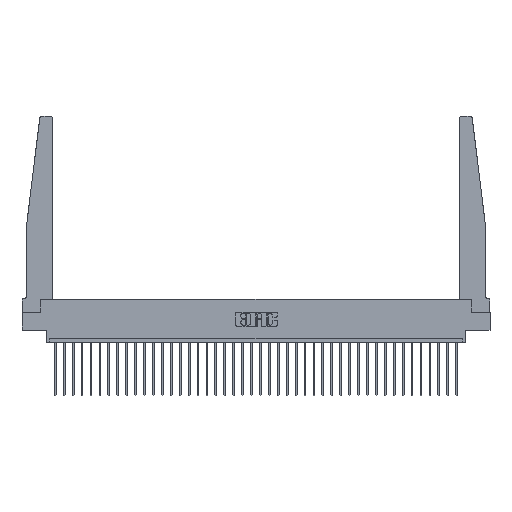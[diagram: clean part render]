
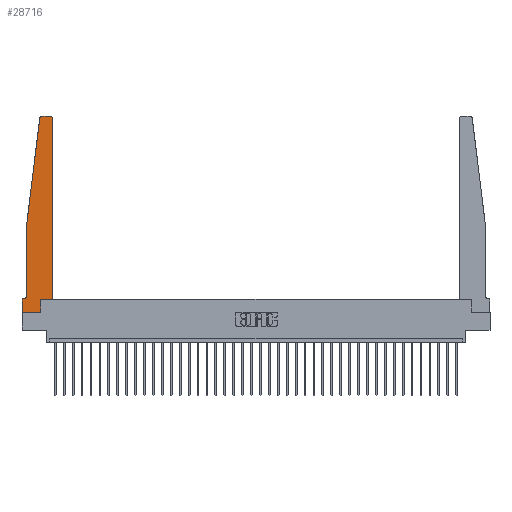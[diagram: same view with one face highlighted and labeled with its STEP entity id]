
A CAD part, top view. The second image highlights one B-rep face of the part: STEP entity #28716.
In plain terms, the highlighted planar face has unit normal (0, 0, 1).
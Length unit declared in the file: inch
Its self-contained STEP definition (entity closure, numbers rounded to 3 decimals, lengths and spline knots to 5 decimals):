
#335 = FACE_OUTER_BOUND ( 'NONE', #23905, .T. ) ;
#540 = AXIS2_PLACEMENT_3D ( 'NONE', #12960, #15313, #5533 ) ;
#733 = DIRECTION ( 'NONE',  ( 0., 0., 1. ) ) ;
#760 = CARTESIAN_POINT ( 'NONE',  ( 0.425, 2.72, 0.37 ) ) ;
#1057 = CIRCLE ( 'NONE', #30986, 0.03 ) ;
#1431 = LINE ( 'NONE', #20981, #18172 ) ;
#2554 = EDGE_CURVE ( 'NONE', #20029, #25679, #28582, .T. ) ;
#2625 = ORIENTED_EDGE ( 'NONE', *, *, #18938, .T. ) ;
#2832 = EDGE_CURVE ( 'NONE', #27348, #9803, #18638, .T. ) ;
#3004 = ORIENTED_EDGE ( 'NONE', *, *, #28220, .T. ) ;
#3468 = DIRECTION ( 'NONE',  ( 1., 0., 0. ) ) ;
#3637 = CARTESIAN_POINT ( 'NONE',  ( 0.27653, 2.72, 0.37 ) ) ;
#5130 = CARTESIAN_POINT ( 'NONE',  ( 0., 0., 0.37 ) ) ;
#5533 = DIRECTION ( 'NONE',  ( 1., 0., 0. ) ) ;
#5964 = CARTESIAN_POINT ( 'NONE',  ( 0.015, 0.1875, 0.37 ) ) ;
#6322 = LINE ( 'NONE', #21762, #27006 ) ;
#6409 = EDGE_CURVE ( 'NONE', #17926, #22845, #7710, .T. ) ;
#6859 = CARTESIAN_POINT ( 'NONE',  ( 0.425, 0.18, 0.37 ) ) ;
#7710 = LINE ( 'NONE', #22271, #25174 ) ;
#8232 = CARTESIAN_POINT ( 'NONE',  ( 0.065, 1.25, 0.37 ) ) ;
#9803 = VERTEX_POINT ( 'NONE', #13535 ) ;
#10226 = CARTESIAN_POINT ( 'NONE',  ( 0.065, 1.25, 0.37 ) ) ;
#10941 = AXIS2_PLACEMENT_3D ( 'NONE', #11388, #13925, #31398 ) ;
#11077 = CIRCLE ( 'NONE', #540, 0.03 ) ;
#11388 = CARTESIAN_POINT ( 'NONE',  ( 0., 0.1875, 0.37 ) ) ;
#11432 = VECTOR ( 'NONE', #13200, 39.37008 ) ;
#11489 = ORIENTED_EDGE ( 'NONE', *, *, #2554, .T. ) ;
#12028 = EDGE_CURVE ( 'NONE', #30605, #20029, #18039, .T. ) ;
#12380 = EDGE_CURVE ( 'NONE', #20665, #26768, #23200, .T. ) ;
#12960 = CARTESIAN_POINT ( 'NONE',  ( 0.395, 2.72, 0.37 ) ) ;
#13132 = CARTESIAN_POINT ( 'NONE',  ( 0.065, 0.2375, 0.37 ) ) ;
#13200 = DIRECTION ( 'NONE',  ( -0.122, -0.992, 0. ) ) ;
#13500 = PLANE ( 'NONE',  #10941 ) ;
#13535 = CARTESIAN_POINT ( 'NONE',  ( 0.2605, 0., 0.37 ) ) ;
#13925 = DIRECTION ( 'NONE',  ( 0., 0., 1. ) ) ;
#14068 = VERTEX_POINT ( 'NONE', #30506 ) ;
#14333 = ORIENTED_EDGE ( 'NONE', *, *, #16728, .T. ) ;
#14335 = AXIS2_PLACEMENT_3D ( 'NONE', #25271, #23043, #20587 ) ;
#15313 = DIRECTION ( 'NONE',  ( 0., 0., 1. ) ) ;
#15903 = ORIENTED_EDGE ( 'NONE', *, *, #17923, .T. ) ;
#16623 = CARTESIAN_POINT ( 'NONE',  ( 0.27653, 2.75, 0.37 ) ) ;
#16728 = EDGE_CURVE ( 'NONE', #25679, #22465, #11077, .T. ) ;
#17233 = VECTOR ( 'NONE', #28024, 39.37008 ) ;
#17825 = CIRCLE ( 'NONE', #14335, 0.05 ) ;
#17841 = VECTOR ( 'NONE', #3468, 39.37008 ) ;
#17923 = EDGE_CURVE ( 'NONE', #22465, #22476, #1431, .T. ) ;
#17926 = VERTEX_POINT ( 'NONE', #5964 ) ;
#18039 = LINE ( 'NONE', #6859, #18835 ) ;
#18124 = CARTESIAN_POINT ( 'NONE',  ( 0.065, 1.25, 0.37 ) ) ;
#18172 = VECTOR ( 'NONE', #21430, 39.37008 ) ;
#18638 = LINE ( 'NONE', #31359, #17841 ) ;
#18835 = VECTOR ( 'NONE', #24525, 39.37008 ) ;
#18938 = EDGE_CURVE ( 'NONE', #14068, #20665, #28979, .T. ) ;
#18998 = DIRECTION ( 'NONE',  ( 0., -1., 0. ) ) ;
#19973 = VECTOR ( 'NONE', #31827, 39.37008 ) ;
#20029 = VERTEX_POINT ( 'NONE', #23597 ) ;
#20587 = DIRECTION ( 'NONE',  ( -1., 0., 0. ) ) ;
#20665 = VERTEX_POINT ( 'NONE', #18124 ) ;
#20981 = CARTESIAN_POINT ( 'NONE',  ( 0.25, 2.75, 0.37 ) ) ;
#21056 = CARTESIAN_POINT ( 'NONE',  ( 0., 0.1875, 0.37 ) ) ;
#21094 = DIRECTION ( 'NONE',  ( 1., 0., 0. ) ) ;
#21430 = DIRECTION ( 'NONE',  ( -1., 0., 0. ) ) ;
#21583 = ORIENTED_EDGE ( 'NONE', *, *, #26490, .T. ) ;
#21728 = CARTESIAN_POINT ( 'NONE',  ( 0.395, 2.75, 0.37 ) ) ;
#21762 = CARTESIAN_POINT ( 'NONE',  ( 0., 0., 0.37 ) ) ;
#22271 = CARTESIAN_POINT ( 'NONE',  ( 0.065, 0.1875, 0.37 ) ) ;
#22465 = VERTEX_POINT ( 'NONE', #21728 ) ;
#22476 = VERTEX_POINT ( 'NONE', #16623 ) ;
#22650 = EDGE_CURVE ( 'NONE', #22476, #14068, #1057, .T. ) ;
#22845 = VERTEX_POINT ( 'NONE', #21056 ) ;
#23043 = DIRECTION ( 'NONE',  ( 0., 0., -1. ) ) ;
#23200 = LINE ( 'NONE', #10226, #17233 ) ;
#23597 = CARTESIAN_POINT ( 'NONE',  ( 0.425, 0.18, 0.37 ) ) ;
#23905 = EDGE_LOOP ( 'NONE', ( #15903, #28594, #2625, #26828, #29696, #32265, #3004, #31463, #21583, #25131, #11489, #14333 ) ) ;
#24388 = CARTESIAN_POINT ( 'NONE',  ( 0.2605, 0.18, 0.37 ) ) ;
#24525 = DIRECTION ( 'NONE',  ( 1., 0., 0. ) ) ;
#25131 = ORIENTED_EDGE ( 'NONE', *, *, #12028, .T. ) ;
#25174 = VECTOR ( 'NONE', #27379, 39.37008 ) ;
#25271 = CARTESIAN_POINT ( 'NONE',  ( 0.015, 0.2375, 0.37 ) ) ;
#25395 = CARTESIAN_POINT ( 'NONE',  ( 0.2605, 0.18, 0.37 ) ) ;
#25679 = VERTEX_POINT ( 'NONE', #760 ) ;
#26490 = EDGE_CURVE ( 'NONE', #9803, #30605, #26746, .T. ) ;
#26556 = VECTOR ( 'NONE', #31367, 39.37008 ) ;
#26746 = LINE ( 'NONE', #24388, #19973 ) ;
#26768 = VERTEX_POINT ( 'NONE', #13132 ) ;
#26828 = ORIENTED_EDGE ( 'NONE', *, *, #12380, .T. ) ;
#27006 = VECTOR ( 'NONE', #18998, 39.37008 ) ;
#27348 = VERTEX_POINT ( 'NONE', #5130 ) ;
#27379 = DIRECTION ( 'NONE',  ( -1., 0., 0. ) ) ;
#28024 = DIRECTION ( 'NONE',  ( 0., -1., 0. ) ) ;
#28220 = EDGE_CURVE ( 'NONE', #22845, #27348, #6322, .T. ) ;
#28582 = LINE ( 'NONE', #28746, #26556 ) ;
#28594 = ORIENTED_EDGE ( 'NONE', *, *, #22650, .T. ) ;
#28716 = ADVANCED_FACE ( 'NONE', ( #335 ), #13500, .T. ) ;
#28746 = CARTESIAN_POINT ( 'NONE',  ( 0.425, 0.18, 0.37 ) ) ;
#28979 = LINE ( 'NONE', #8232, #11432 ) ;
#29114 = EDGE_CURVE ( 'NONE', #26768, #17926, #17825, .T. ) ;
#29696 = ORIENTED_EDGE ( 'NONE', *, *, #29114, .T. ) ;
#30506 = CARTESIAN_POINT ( 'NONE',  ( 0.24675, 2.72367, 0.37 ) ) ;
#30605 = VERTEX_POINT ( 'NONE', #25395 ) ;
#30986 = AXIS2_PLACEMENT_3D ( 'NONE', #3637, #733, #21094 ) ;
#31359 = CARTESIAN_POINT ( 'NONE',  ( 0., 0., 0.37 ) ) ;
#31367 = DIRECTION ( 'NONE',  ( 0., 1., 0. ) ) ;
#31398 = DIRECTION ( 'NONE',  ( 1., 0., 0. ) ) ;
#31463 = ORIENTED_EDGE ( 'NONE', *, *, #2832, .T. ) ;
#31827 = DIRECTION ( 'NONE',  ( 0., 1., 0. ) ) ;
#32265 = ORIENTED_EDGE ( 'NONE', *, *, #6409, .T. ) ;
